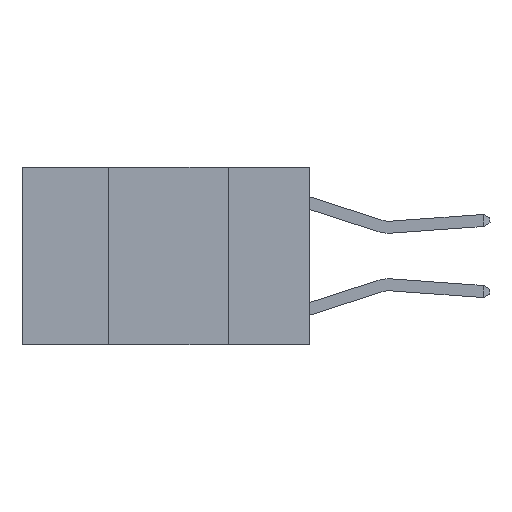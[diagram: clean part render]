
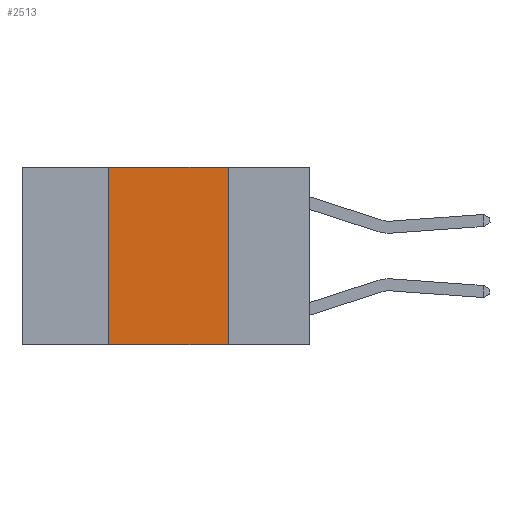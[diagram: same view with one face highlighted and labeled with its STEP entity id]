
A CAD part, left-side view. The second image highlights one B-rep face of the part: STEP entity #2513.
In plain terms, the highlighted planar face has unit normal (-1, 0, 0).
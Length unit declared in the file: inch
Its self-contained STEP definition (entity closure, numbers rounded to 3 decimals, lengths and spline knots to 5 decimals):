
#318 = CARTESIAN_POINT ( 'NONE',  ( 0., 0.17, 0. ) ) ;
#794 = ORIENTED_EDGE ( 'NONE', *, *, #16306, .F. ) ;
#815 = VECTOR ( 'NONE', #23342, 39.37008 ) ;
#2469 = LINE ( 'NONE', #318, #23217 ) ;
#2513 = ADVANCED_FACE ( 'NONE', ( #20437 ), #15352, .F. ) ;
#2923 = VECTOR ( 'NONE', #21008, 39.37008 ) ;
#3674 = CARTESIAN_POINT ( 'NONE',  ( 0., 0.6, 0. ) ) ;
#4182 = ORIENTED_EDGE ( 'NONE', *, *, #13326, .F. ) ;
#4555 = EDGE_CURVE ( 'NONE', #23145, #8630, #20938, .T. ) ;
#5624 = DIRECTION ( 'NONE',  ( 1., 0., 0. ) ) ;
#8319 = ORIENTED_EDGE ( 'NONE', *, *, #11069, .F. ) ;
#8630 = VERTEX_POINT ( 'NONE', #17827 ) ;
#9694 = CARTESIAN_POINT ( 'NONE',  ( 0., 0.6, -0.37 ) ) ;
#10760 = CARTESIAN_POINT ( 'NONE',  ( 0., 0.17, 0. ) ) ;
#10896 = EDGE_LOOP ( 'NONE', ( #794, #4182, #8319, #23979 ) ) ;
#11069 = EDGE_CURVE ( 'NONE', #23145, #20290, #13288, .T. ) ;
#13288 = LINE ( 'NONE', #24908, #2923 ) ;
#13326 = EDGE_CURVE ( 'NONE', #20290, #21801, #17530, .T. ) ;
#13936 = DIRECTION ( 'NONE',  ( 0., 0., -1. ) ) ;
#14967 = CARTESIAN_POINT ( 'NONE',  ( 0., 0.6, 0. ) ) ;
#15352 = PLANE ( 'NONE',  #16547 ) ;
#16306 = EDGE_CURVE ( 'NONE', #21801, #8630, #2469, .T. ) ;
#16547 = AXIS2_PLACEMENT_3D ( 'NONE', #3674, #5624, #19268 ) ;
#16916 = VECTOR ( 'NONE', #16938, 39.37008 ) ;
#16938 = DIRECTION ( 'NONE',  ( 0., -1., 0. ) ) ;
#17530 = LINE ( 'NONE', #14967, #16916 ) ;
#17827 = CARTESIAN_POINT ( 'NONE',  ( 0., 0.17, -0.37 ) ) ;
#18100 = CARTESIAN_POINT ( 'NONE',  ( 0., 0.42, 0. ) ) ;
#19268 = DIRECTION ( 'NONE',  ( 0., 0., -1. ) ) ;
#19709 = CARTESIAN_POINT ( 'NONE',  ( 0., 0.42, -0.37 ) ) ;
#20290 = VERTEX_POINT ( 'NONE', #18100 ) ;
#20437 = FACE_OUTER_BOUND ( 'NONE', #10896, .T. ) ;
#20938 = LINE ( 'NONE', #9694, #815 ) ;
#21008 = DIRECTION ( 'NONE',  ( 0., 0., 1. ) ) ;
#21801 = VERTEX_POINT ( 'NONE', #10760 ) ;
#23145 = VERTEX_POINT ( 'NONE', #19709 ) ;
#23217 = VECTOR ( 'NONE', #13936, 39.37008 ) ;
#23342 = DIRECTION ( 'NONE',  ( 0., -1., 0. ) ) ;
#23979 = ORIENTED_EDGE ( 'NONE', *, *, #4555, .T. ) ;
#24908 = CARTESIAN_POINT ( 'NONE',  ( 0., 0.42, 0. ) ) ;
